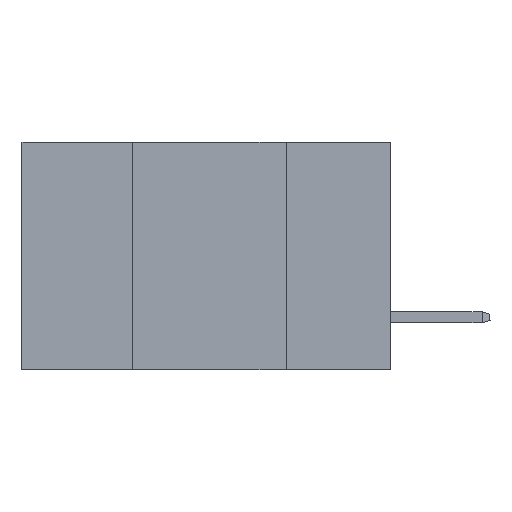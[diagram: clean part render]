
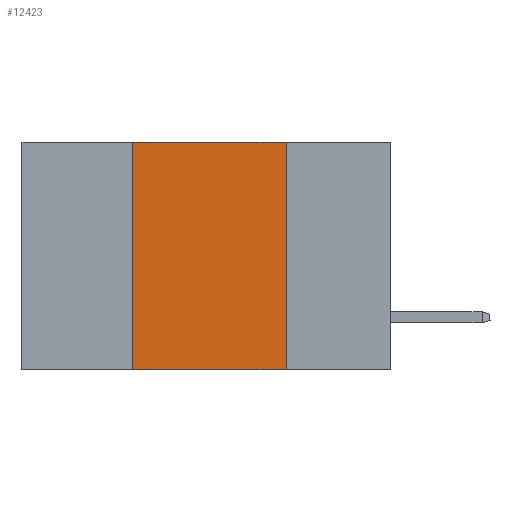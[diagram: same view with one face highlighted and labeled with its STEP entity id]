
A CAD part, left-side view. The second image highlights one B-rep face of the part: STEP entity #12423.
In plain terms, the highlighted planar face has unit normal (-1, 0, 0).
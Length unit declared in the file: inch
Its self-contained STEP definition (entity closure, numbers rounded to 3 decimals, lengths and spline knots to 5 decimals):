
#70 = DIRECTION ( 'NONE',  ( 0., -1., 0. ) ) ;
#268 = LINE ( 'NONE', #3822, #8503 ) ;
#541 = CARTESIAN_POINT ( 'NONE',  ( 0., 0.17, 0. ) ) ;
#813 = FACE_OUTER_BOUND ( 'NONE', #20866, .T. ) ;
#1449 = CARTESIAN_POINT ( 'NONE',  ( 0., 0.6, -0.37 ) ) ;
#2217 = LINE ( 'NONE', #12293, #10409 ) ;
#2388 = DIRECTION ( 'NONE',  ( 0., 0., -1. ) ) ;
#2421 = VECTOR ( 'NONE', #6495, 39.37008 ) ;
#3822 = CARTESIAN_POINT ( 'NONE',  ( 0., 0.17, 0. ) ) ;
#4295 = EDGE_CURVE ( 'NONE', #6508, #16542, #2217, .T. ) ;
#4936 = ORIENTED_EDGE ( 'NONE', *, *, #14416, .F. ) ;
#5372 = EDGE_CURVE ( 'NONE', #6508, #6273, #15532, .T. ) ;
#5701 = ORIENTED_EDGE ( 'NONE', *, *, #5372, .T. ) ;
#5907 = CARTESIAN_POINT ( 'NONE',  ( 0., 0.17, -0.37 ) ) ;
#6188 = VECTOR ( 'NONE', #70, 39.37008 ) ;
#6273 = VERTEX_POINT ( 'NONE', #5907 ) ;
#6495 = DIRECTION ( 'NONE',  ( 0., -1., 0. ) ) ;
#6508 = VERTEX_POINT ( 'NONE', #11796 ) ;
#6562 = CARTESIAN_POINT ( 'NONE',  ( 0., 0.6, 0. ) ) ;
#7111 = DIRECTION ( 'NONE',  ( 1., 0., 0. ) ) ;
#7184 = PLANE ( 'NONE',  #19865 ) ;
#8503 = VECTOR ( 'NONE', #15469, 39.37008 ) ;
#8693 = CARTESIAN_POINT ( 'NONE',  ( 0., 0.6, 0. ) ) ;
#9788 = ORIENTED_EDGE ( 'NONE', *, *, #20015, .F. ) ;
#10409 = VECTOR ( 'NONE', #18178, 39.37008 ) ;
#10565 = LINE ( 'NONE', #6562, #6188 ) ;
#11050 = VERTEX_POINT ( 'NONE', #541 ) ;
#11796 = CARTESIAN_POINT ( 'NONE',  ( 0., 0.42, -0.37 ) ) ;
#12293 = CARTESIAN_POINT ( 'NONE',  ( 0., 0.42, 0. ) ) ;
#12423 = ADVANCED_FACE ( 'NONE', ( #813 ), #7184, .F. ) ;
#13864 = ORIENTED_EDGE ( 'NONE', *, *, #4295, .F. ) ;
#14416 = EDGE_CURVE ( 'NONE', #16542, #11050, #10565, .T. ) ;
#15469 = DIRECTION ( 'NONE',  ( 0., 0., -1. ) ) ;
#15532 = LINE ( 'NONE', #1449, #2421 ) ;
#16542 = VERTEX_POINT ( 'NONE', #18515 ) ;
#18178 = DIRECTION ( 'NONE',  ( 0., 0., 1. ) ) ;
#18515 = CARTESIAN_POINT ( 'NONE',  ( 0., 0.42, 0. ) ) ;
#19865 = AXIS2_PLACEMENT_3D ( 'NONE', #8693, #7111, #2388 ) ;
#20015 = EDGE_CURVE ( 'NONE', #11050, #6273, #268, .T. ) ;
#20866 = EDGE_LOOP ( 'NONE', ( #9788, #4936, #13864, #5701 ) ) ;
